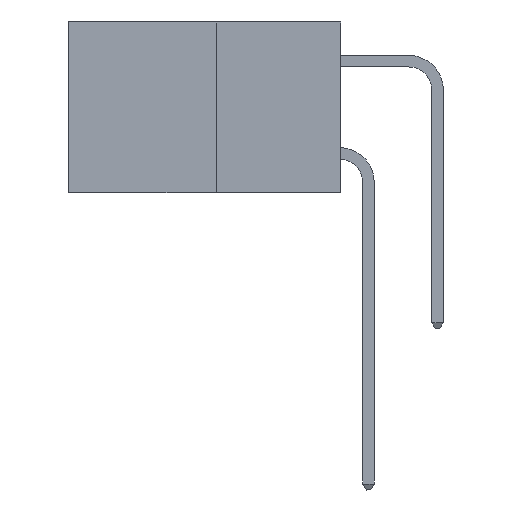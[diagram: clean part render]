
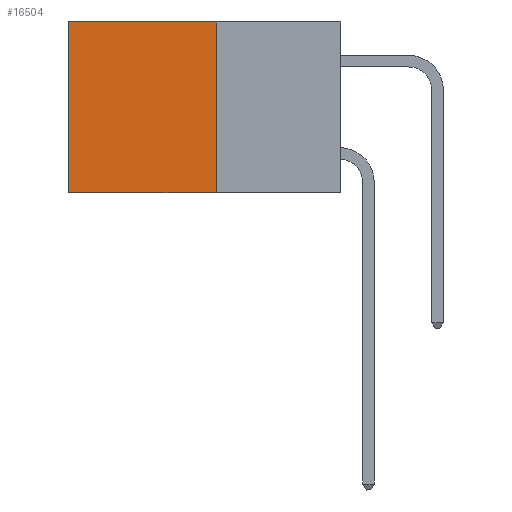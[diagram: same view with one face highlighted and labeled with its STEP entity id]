
A CAD part, left-side view. The second image highlights one B-rep face of the part: STEP entity #16504.
In plain terms, the highlighted planar face has unit normal (-1, 0, 0).
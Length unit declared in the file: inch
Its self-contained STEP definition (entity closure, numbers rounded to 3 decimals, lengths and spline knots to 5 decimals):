
#168 = CARTESIAN_POINT ( 'NONE',  ( 0.277, 0.27, -0.37 ) ) ;
#353 = VERTEX_POINT ( 'NONE', #4862 ) ;
#1482 = DIRECTION ( 'NONE',  ( 0., 1., 0. ) ) ;
#1495 = AXIS2_PLACEMENT_3D ( 'NONE', #168, #16666, #5724 ) ;
#2596 = LINE ( 'NONE', #3430, #11803 ) ;
#3119 = DIRECTION ( 'NONE',  ( 0., 0., -1. ) ) ;
#3430 = CARTESIAN_POINT ( 'NONE',  ( 0.277, 0.27, -0.37 ) ) ;
#3882 = PLANE ( 'NONE',  #1495 ) ;
#4418 = FACE_OUTER_BOUND ( 'NONE', #22867, .T. ) ;
#4827 = EDGE_CURVE ( 'NONE', #16789, #353, #21145, .T. ) ;
#4862 = CARTESIAN_POINT ( 'NONE',  ( 0.277, 0.59, 0. ) ) ;
#5724 = DIRECTION ( 'NONE',  ( 0., 0., -1. ) ) ;
#6133 = LINE ( 'NONE', #23264, #15262 ) ;
#6897 = DIRECTION ( 'NONE',  ( 0., 0., -1. ) ) ;
#6981 = VERTEX_POINT ( 'NONE', #15035 ) ;
#7275 = EDGE_CURVE ( 'NONE', #16789, #14668, #2596, .T. ) ;
#8272 = CARTESIAN_POINT ( 'NONE',  ( 0.277, 0.27, 0. ) ) ;
#10567 = VECTOR ( 'NONE', #6897, 39.37008 ) ;
#11113 = LINE ( 'NONE', #17734, #10567 ) ;
#11803 = VECTOR ( 'NONE', #3119, 39.37008 ) ;
#13638 = CARTESIAN_POINT ( 'NONE',  ( 0.277, 0.27, -0.37 ) ) ;
#14668 = VERTEX_POINT ( 'NONE', #13638 ) ;
#15035 = CARTESIAN_POINT ( 'NONE',  ( 0.277, 0.59, -0.37 ) ) ;
#15262 = VECTOR ( 'NONE', #1482, 39.37008 ) ;
#15547 = EDGE_CURVE ( 'NONE', #353, #6981, #11113, .T. ) ;
#16193 = ORIENTED_EDGE ( 'NONE', *, *, #7275, .F. ) ;
#16363 = VECTOR ( 'NONE', #16799, 39.37008 ) ;
#16504 = ADVANCED_FACE ( 'NONE', ( #4418 ), #3882, .F. ) ;
#16666 = DIRECTION ( 'NONE',  ( 1., 0., 0. ) ) ;
#16789 = VERTEX_POINT ( 'NONE', #8272 ) ;
#16799 = DIRECTION ( 'NONE',  ( 0., 1., 0. ) ) ;
#17300 = CARTESIAN_POINT ( 'NONE',  ( 0.277, 0.27, 0. ) ) ;
#17383 = ORIENTED_EDGE ( 'NONE', *, *, #19272, .F. ) ;
#17734 = CARTESIAN_POINT ( 'NONE',  ( 0.277, 0.59, -0.37 ) ) ;
#19272 = EDGE_CURVE ( 'NONE', #14668, #6981, #6133, .T. ) ;
#20611 = ORIENTED_EDGE ( 'NONE', *, *, #15547, .T. ) ;
#21145 = LINE ( 'NONE', #17300, #16363 ) ;
#22867 = EDGE_LOOP ( 'NONE', ( #20611, #17383, #16193, #23294 ) ) ;
#23264 = CARTESIAN_POINT ( 'NONE',  ( 0.277, 0.27, -0.37 ) ) ;
#23294 = ORIENTED_EDGE ( 'NONE', *, *, #4827, .T. ) ;
